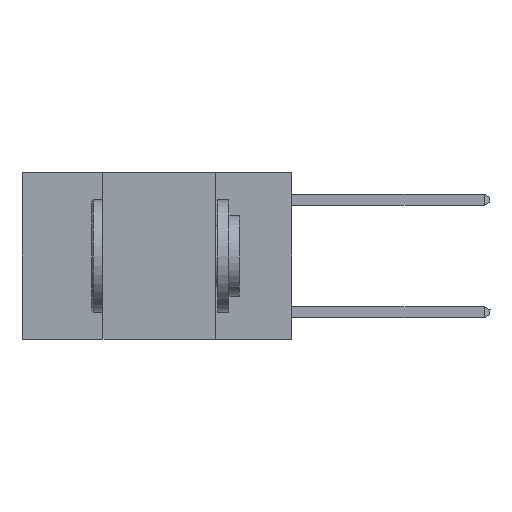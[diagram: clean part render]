
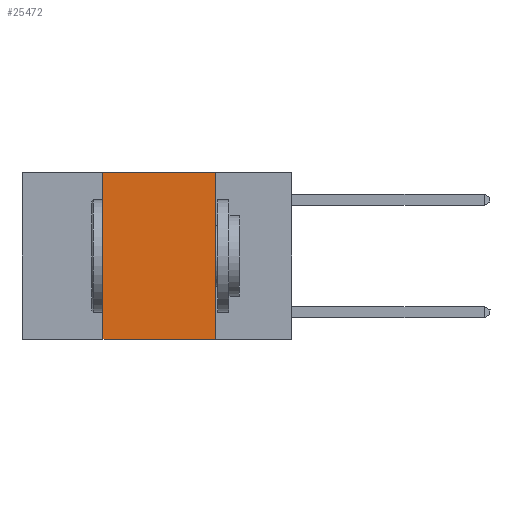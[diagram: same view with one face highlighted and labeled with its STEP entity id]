
A CAD part, left-side view. The second image highlights one B-rep face of the part: STEP entity #25472.
In plain terms, the highlighted planar face has unit normal (-1, 0, 0).
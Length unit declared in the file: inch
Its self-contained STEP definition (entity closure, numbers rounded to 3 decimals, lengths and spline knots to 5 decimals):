
#343 = DIRECTION ( 'NONE',  ( 0., 0., -1. ) ) ;
#890 = DIRECTION ( 'NONE',  ( 0., 0., -1. ) ) ;
#2663 = CARTESIAN_POINT ( 'NONE',  ( 0., 0.6, -0.37 ) ) ;
#3133 = VERTEX_POINT ( 'NONE', #4990 ) ;
#4571 = DIRECTION ( 'NONE',  ( 0., 0., 1. ) ) ;
#4990 = CARTESIAN_POINT ( 'NONE',  ( 0., 0.42, -0.37 ) ) ;
#4997 = VECTOR ( 'NONE', #4571, 39.37008 ) ;
#5440 = VECTOR ( 'NONE', #14935, 39.37008 ) ;
#5911 = VECTOR ( 'NONE', #26481, 39.37008 ) ;
#6250 = LINE ( 'NONE', #2663, #5440 ) ;
#6547 = EDGE_CURVE ( 'NONE', #3133, #30686, #6250, .T. ) ;
#8326 = PLANE ( 'NONE',  #12177 ) ;
#8638 = ORIENTED_EDGE ( 'NONE', *, *, #11523, .F. ) ;
#9676 = ORIENTED_EDGE ( 'NONE', *, *, #22171, .F. ) ;
#9851 = EDGE_CURVE ( 'NONE', #3133, #29906, #24467, .T. ) ;
#9989 = ORIENTED_EDGE ( 'NONE', *, *, #9851, .F. ) ;
#10624 = ORIENTED_EDGE ( 'NONE', *, *, #6547, .T. ) ;
#11523 = EDGE_CURVE ( 'NONE', #29795, #30686, #16793, .T. ) ;
#12177 = AXIS2_PLACEMENT_3D ( 'NONE', #29929, #15677, #890 ) ;
#12595 = CARTESIAN_POINT ( 'NONE',  ( 0., 0.42, 0. ) ) ;
#12969 = EDGE_LOOP ( 'NONE', ( #8638, #9676, #9989, #10624 ) ) ;
#13989 = LINE ( 'NONE', #30982, #5911 ) ;
#14935 = DIRECTION ( 'NONE',  ( 0., -1., 0. ) ) ;
#15677 = DIRECTION ( 'NONE',  ( 1., 0., 0. ) ) ;
#16793 = LINE ( 'NONE', #17562, #22465 ) ;
#16948 = CARTESIAN_POINT ( 'NONE',  ( 0., 0.17, 0. ) ) ;
#17562 = CARTESIAN_POINT ( 'NONE',  ( 0., 0.17, 0. ) ) ;
#20615 = CARTESIAN_POINT ( 'NONE',  ( 0., 0.17, -0.37 ) ) ;
#22171 = EDGE_CURVE ( 'NONE', #29906, #29795, #13989, .T. ) ;
#22465 = VECTOR ( 'NONE', #343, 39.37008 ) ;
#22518 = FACE_OUTER_BOUND ( 'NONE', #12969, .T. ) ;
#24467 = LINE ( 'NONE', #31017, #4997 ) ;
#25472 = ADVANCED_FACE ( 'NONE', ( #22518 ), #8326, .F. ) ;
#26481 = DIRECTION ( 'NONE',  ( 0., -1., 0. ) ) ;
#29795 = VERTEX_POINT ( 'NONE', #16948 ) ;
#29906 = VERTEX_POINT ( 'NONE', #12595 ) ;
#29929 = CARTESIAN_POINT ( 'NONE',  ( 0., 0.6, 0. ) ) ;
#30686 = VERTEX_POINT ( 'NONE', #20615 ) ;
#30982 = CARTESIAN_POINT ( 'NONE',  ( 0., 0.6, 0. ) ) ;
#31017 = CARTESIAN_POINT ( 'NONE',  ( 0., 0.42, 0. ) ) ;
